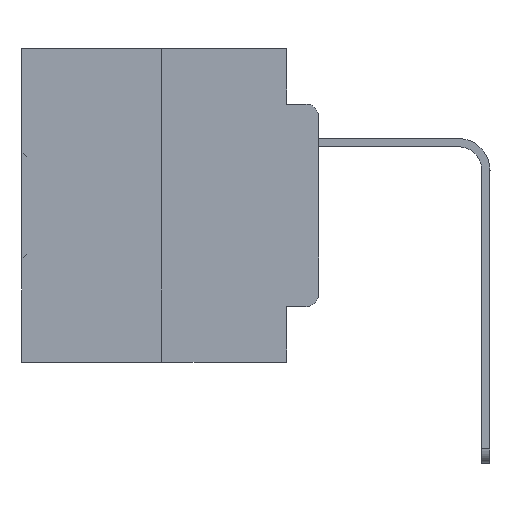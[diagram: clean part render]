
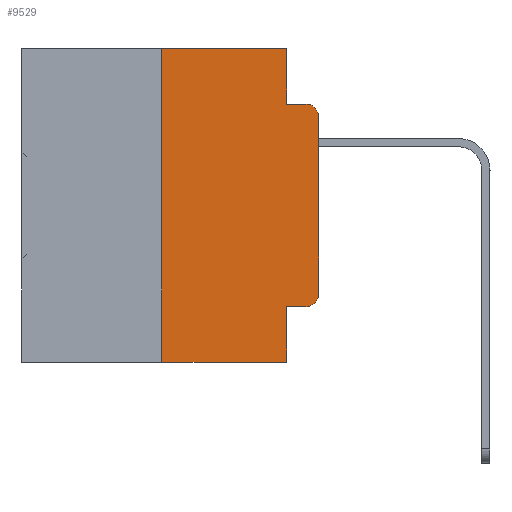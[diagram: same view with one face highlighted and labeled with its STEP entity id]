
A CAD part, left-side view. The second image highlights one B-rep face of the part: STEP entity #9529.
In plain terms, the highlighted planar face has unit normal (-1, 0, 0).
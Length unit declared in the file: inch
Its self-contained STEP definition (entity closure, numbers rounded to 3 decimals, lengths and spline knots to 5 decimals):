
#579 = VECTOR ( 'NONE', #29475, 39.37008 ) ;
#1094 = VERTEX_POINT ( 'NONE', #17092 ) ;
#1117 = CARTESIAN_POINT ( 'NONE',  ( 0., 0.051, -0.4115 ) ) ;
#1991 = CARTESIAN_POINT ( 'NONE',  ( 0., 0.02, -0.0885 ) ) ;
#2068 = VECTOR ( 'NONE', #15000, 39.37008 ) ;
#2139 = LINE ( 'NONE', #22019, #26098 ) ;
#2158 = CIRCLE ( 'NONE', #31044, 0.02 ) ;
#3125 = DIRECTION ( 'NONE',  ( -1., 0., 0. ) ) ;
#3397 = CARTESIAN_POINT ( 'NONE',  ( 0., 0.473, 0. ) ) ;
#3666 = EDGE_CURVE ( 'NONE', #7106, #17299, #21959, .T. ) ;
#4063 = VERTEX_POINT ( 'NONE', #1117 ) ;
#5174 = CARTESIAN_POINT ( 'NONE',  ( 0., 0.02, -0.4115 ) ) ;
#5621 = CARTESIAN_POINT ( 'NONE',  ( 0., 0.25, 0. ) ) ;
#5863 = VERTEX_POINT ( 'NONE', #1991 ) ;
#5934 = LINE ( 'NONE', #17587, #9994 ) ;
#6298 = DIRECTION ( 'NONE',  ( 0., 0., -1. ) ) ;
#6305 = ORIENTED_EDGE ( 'NONE', *, *, #32100, .F. ) ;
#6508 = DIRECTION ( 'NONE',  ( 0., -1., 0. ) ) ;
#6572 = AXIS2_PLACEMENT_3D ( 'NONE', #23337, #31153, #26172 ) ;
#6726 = CARTESIAN_POINT ( 'NONE',  ( 0., 0.051, -0.4115 ) ) ;
#7009 = VERTEX_POINT ( 'NONE', #27679 ) ;
#7019 = LINE ( 'NONE', #9244, #16370 ) ;
#7106 = VERTEX_POINT ( 'NONE', #7222 ) ;
#7222 = CARTESIAN_POINT ( 'NONE',  ( 0., 0., -0.3915 ) ) ;
#7523 = VECTOR ( 'NONE', #6508, 39.37008 ) ;
#7915 = DIRECTION ( 'NONE',  ( 0., 0., 1. ) ) ;
#9197 = VECTOR ( 'NONE', #7915, 39.37008 ) ;
#9234 = CARTESIAN_POINT ( 'NONE',  ( 0., 0.051, -0.5 ) ) ;
#9244 = CARTESIAN_POINT ( 'NONE',  ( 0., 0.051, -0.0885 ) ) ;
#9253 = VERTEX_POINT ( 'NONE', #14406 ) ;
#9529 = ADVANCED_FACE ( 'NONE', ( #15779 ), #10268, .F. ) ;
#9994 = VECTOR ( 'NONE', #33262, 39.37008 ) ;
#10268 = PLANE ( 'NONE',  #6572 ) ;
#11042 = EDGE_CURVE ( 'NONE', #4063, #29933, #22971, .T. ) ;
#11684 = DIRECTION ( 'NONE',  ( 0., 0., -1. ) ) ;
#11843 = CARTESIAN_POINT ( 'NONE',  ( 0., 0.051, 0. ) ) ;
#12636 = ORIENTED_EDGE ( 'NONE', *, *, #16249, .F. ) ;
#12985 = VECTOR ( 'NONE', #19314, 39.37008 ) ;
#14133 = VERTEX_POINT ( 'NONE', #5621 ) ;
#14406 = CARTESIAN_POINT ( 'NONE',  ( 0., 0.051, -0.0885 ) ) ;
#14983 = EDGE_CURVE ( 'NONE', #4063, #19043, #2139, .T. ) ;
#15000 = DIRECTION ( 'NONE',  ( 0., 0., 1. ) ) ;
#15207 = LINE ( 'NONE', #3397, #579 ) ;
#15779 = FACE_OUTER_BOUND ( 'NONE', #16947, .T. ) ;
#16249 = EDGE_CURVE ( 'NONE', #7009, #9253, #29648, .T. ) ;
#16370 = VECTOR ( 'NONE', #27423, 39.37008 ) ;
#16560 = ORIENTED_EDGE ( 'NONE', *, *, #18096, .F. ) ;
#16607 = ORIENTED_EDGE ( 'NONE', *, *, #18028, .T. ) ;
#16947 = EDGE_LOOP ( 'NONE', ( #21506, #25445, #6305, #12636, #24013, #16560, #16607, #21678, #28376, #22213 ) ) ;
#17092 = CARTESIAN_POINT ( 'NONE',  ( 0., 0.25, -0.5 ) ) ;
#17171 = CARTESIAN_POINT ( 'NONE',  ( 0., 0., -0.1085 ) ) ;
#17299 = VERTEX_POINT ( 'NONE', #17171 ) ;
#17587 = CARTESIAN_POINT ( 'NONE',  ( 0., 0.473, -0.5 ) ) ;
#18028 = EDGE_CURVE ( 'NONE', #1094, #19043, #5934, .T. ) ;
#18096 = EDGE_CURVE ( 'NONE', #1094, #14133, #20985, .T. ) ;
#18630 = CARTESIAN_POINT ( 'NONE',  ( 0., 0.02, -0.3915 ) ) ;
#19043 = VERTEX_POINT ( 'NONE', #9234 ) ;
#19314 = DIRECTION ( 'NONE',  ( 0., 0., -1. ) ) ;
#20985 = LINE ( 'NONE', #28814, #9197 ) ;
#21506 = ORIENTED_EDGE ( 'NONE', *, *, #3666, .T. ) ;
#21678 = ORIENTED_EDGE ( 'NONE', *, *, #14983, .F. ) ;
#21705 = AXIS2_PLACEMENT_3D ( 'NONE', #25375, #22186, #6298 ) ;
#21959 = LINE ( 'NONE', #33587, #2068 ) ;
#22019 = CARTESIAN_POINT ( 'NONE',  ( 0., 0.051, 0. ) ) ;
#22186 = DIRECTION ( 'NONE',  ( -1., 0., 0. ) ) ;
#22213 = ORIENTED_EDGE ( 'NONE', *, *, #26398, .T. ) ;
#22971 = LINE ( 'NONE', #6726, #7523 ) ;
#23337 = CARTESIAN_POINT ( 'NONE',  ( 0., 0.473, 0. ) ) ;
#23878 = DIRECTION ( 'NONE',  ( 0., 0., -1. ) ) ;
#24013 = ORIENTED_EDGE ( 'NONE', *, *, #31359, .F. ) ;
#25375 = CARTESIAN_POINT ( 'NONE',  ( 0., 0.02, -0.1085 ) ) ;
#25445 = ORIENTED_EDGE ( 'NONE', *, *, #26045, .T. ) ;
#26045 = EDGE_CURVE ( 'NONE', #17299, #5863, #27767, .T. ) ;
#26098 = VECTOR ( 'NONE', #11684, 39.37008 ) ;
#26172 = DIRECTION ( 'NONE',  ( 0., 0., -1. ) ) ;
#26398 = EDGE_CURVE ( 'NONE', #29933, #7106, #2158, .T. ) ;
#27423 = DIRECTION ( 'NONE',  ( 0., -1., 0. ) ) ;
#27679 = CARTESIAN_POINT ( 'NONE',  ( 0., 0.051, 0. ) ) ;
#27767 = CIRCLE ( 'NONE', #21705, 0.02 ) ;
#28376 = ORIENTED_EDGE ( 'NONE', *, *, #11042, .T. ) ;
#28814 = CARTESIAN_POINT ( 'NONE',  ( 0., 0.25, 0. ) ) ;
#29475 = DIRECTION ( 'NONE',  ( 0., -1., 0. ) ) ;
#29648 = LINE ( 'NONE', #11843, #12985 ) ;
#29933 = VERTEX_POINT ( 'NONE', #5174 ) ;
#31044 = AXIS2_PLACEMENT_3D ( 'NONE', #18630, #3125, #23878 ) ;
#31153 = DIRECTION ( 'NONE',  ( 1., 0., 0. ) ) ;
#31359 = EDGE_CURVE ( 'NONE', #14133, #7009, #15207, .T. ) ;
#32100 = EDGE_CURVE ( 'NONE', #9253, #5863, #7019, .T. ) ;
#33262 = DIRECTION ( 'NONE',  ( 0., -1., 0. ) ) ;
#33587 = CARTESIAN_POINT ( 'NONE',  ( 0., 0., 0. ) ) ;
